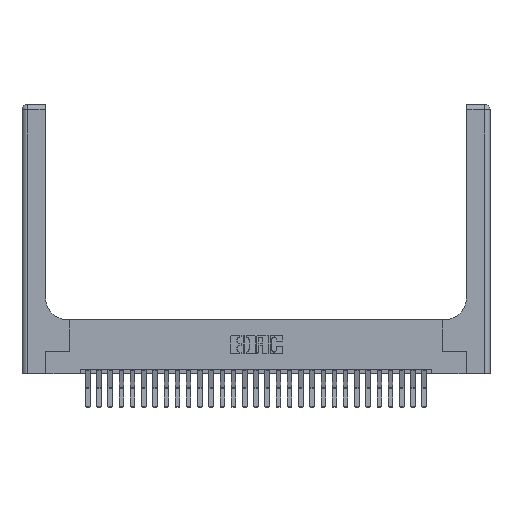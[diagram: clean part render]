
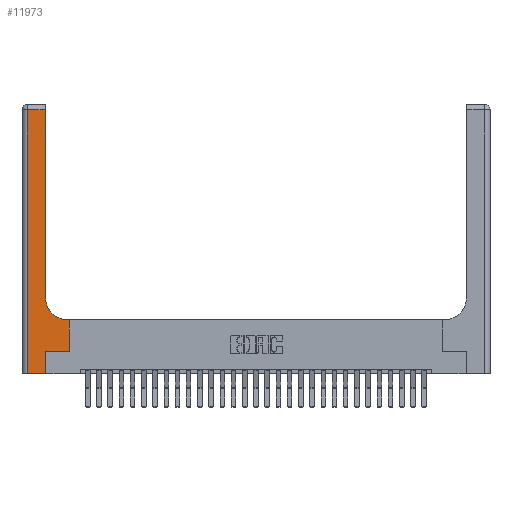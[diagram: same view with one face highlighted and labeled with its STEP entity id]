
A CAD part, top view. The second image highlights one B-rep face of the part: STEP entity #11973.
In plain terms, the highlighted planar face has unit normal (0, 0, 1).
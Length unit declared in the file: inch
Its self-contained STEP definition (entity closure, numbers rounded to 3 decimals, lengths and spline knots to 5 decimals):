
#353 = CARTESIAN_POINT ( 'NONE',  ( 0.26, 0.85, 0.37 ) ) ;
#372 = VECTOR ( 'NONE', #5949, 39.37008 ) ;
#550 = VECTOR ( 'NONE', #26776, 39.37008 ) ;
#918 = DIRECTION ( 'NONE',  ( 0., 1., 0. ) ) ;
#1443 = VECTOR ( 'NONE', #22164, 39.37008 ) ;
#1500 = CARTESIAN_POINT ( 'NONE',  ( 0.528, 0.6, 0.37 ) ) ;
#1703 = CARTESIAN_POINT ( 'NONE',  ( 0.06, 3., 0.37 ) ) ;
#2152 = VECTOR ( 'NONE', #21923, 39.37008 ) ;
#2194 = VERTEX_POINT ( 'NONE', #26470 ) ;
#2475 = VECTOR ( 'NONE', #24193, 39.37008 ) ;
#2741 = FACE_OUTER_BOUND ( 'NONE', #7920, .T. ) ;
#2832 = CARTESIAN_POINT ( 'NONE',  ( 0.528, 0.25, 0.37 ) ) ;
#2916 = CARTESIAN_POINT ( 'NONE',  ( 0., 3., 0.37 ) ) ;
#3122 = LINE ( 'NONE', #1703, #550 ) ;
#3288 = LINE ( 'NONE', #10048, #372 ) ;
#3706 = DIRECTION ( 'NONE',  ( 1., 0., 0. ) ) ;
#3867 = DIRECTION ( 'NONE',  ( 0., 1., 0. ) ) ;
#4148 = VERTEX_POINT ( 'NONE', #10153 ) ;
#4173 = EDGE_CURVE ( 'NONE', #6302, #22928, #17925, .T. ) ;
#4241 = ORIENTED_EDGE ( 'NONE', *, *, #5805, .T. ) ;
#5735 = EDGE_CURVE ( 'NONE', #17416, #2194, #3122, .T. ) ;
#5805 = EDGE_CURVE ( 'NONE', #22795, #18878, #3288, .T. ) ;
#5823 = ORIENTED_EDGE ( 'NONE', *, *, #12052, .T. ) ;
#5924 = CARTESIAN_POINT ( 'NONE',  ( 0.265, 0., 0.37 ) ) ;
#5949 = DIRECTION ( 'NONE',  ( 1., 0., 0. ) ) ;
#6302 = VERTEX_POINT ( 'NONE', #353 ) ;
#6583 = CIRCLE ( 'NONE', #9615, 0.25 ) ;
#6872 = AXIS2_PLACEMENT_3D ( 'NONE', #2916, #17499, #7215 ) ;
#7215 = DIRECTION ( 'NONE',  ( -1., 0., 0. ) ) ;
#7342 = CARTESIAN_POINT ( 'NONE',  ( 0.265, 0., 0.37 ) ) ;
#7920 = EDGE_LOOP ( 'NONE', ( #12587, #22412, #9055, #22798, #24188, #4241, #15621, #5823, #16695 ) ) ;
#7940 = CARTESIAN_POINT ( 'NONE',  ( 0.51, 0.85, 0.37 ) ) ;
#8117 = DIRECTION ( 'NONE',  ( 0., 0., -1. ) ) ;
#8351 = CARTESIAN_POINT ( 'NONE',  ( 0.265, 0.25, 0.37 ) ) ;
#9055 = ORIENTED_EDGE ( 'NONE', *, *, #5735, .T. ) ;
#9591 = EDGE_CURVE ( 'NONE', #4148, #6302, #6583, .T. ) ;
#9615 = AXIS2_PLACEMENT_3D ( 'NONE', #7940, #8117, #22510 ) ;
#10048 = CARTESIAN_POINT ( 'NONE',  ( 0.265, 0.25, 0.37 ) ) ;
#10153 = CARTESIAN_POINT ( 'NONE',  ( 0.51, 0.6, 0.37 ) ) ;
#11111 = EDGE_CURVE ( 'NONE', #18878, #23563, #21078, .T. ) ;
#11221 = EDGE_CURVE ( 'NONE', #12202, #22795, #18783, .T. ) ;
#11266 = CARTESIAN_POINT ( 'NONE',  ( 0.06, 2.94, 0.37 ) ) ;
#11388 = VECTOR ( 'NONE', #3706, 39.37008 ) ;
#11712 = LINE ( 'NONE', #11822, #11388 ) ;
#11822 = CARTESIAN_POINT ( 'NONE',  ( 0., 0., 0.37 ) ) ;
#11973 = ADVANCED_FACE ( 'NONE', ( #2741 ), #23725, .F. ) ;
#12052 = EDGE_CURVE ( 'NONE', #23563, #4148, #14469, .T. ) ;
#12202 = VERTEX_POINT ( 'NONE', #5924 ) ;
#12587 = ORIENTED_EDGE ( 'NONE', *, *, #4173, .T. ) ;
#12695 = CARTESIAN_POINT ( 'NONE',  ( 0.26, 2.94, 0.37 ) ) ;
#13572 = CARTESIAN_POINT ( 'NONE',  ( 0.26, 0.6, 0.37 ) ) ;
#14469 = LINE ( 'NONE', #13572, #1443 ) ;
#15368 = EDGE_CURVE ( 'NONE', #2194, #12202, #11712, .T. ) ;
#15621 = ORIENTED_EDGE ( 'NONE', *, *, #11111, .T. ) ;
#16325 = CARTESIAN_POINT ( 'NONE',  ( 0.26, 3., 0.37 ) ) ;
#16695 = ORIENTED_EDGE ( 'NONE', *, *, #9591, .T. ) ;
#17416 = VERTEX_POINT ( 'NONE', #11266 ) ;
#17499 = DIRECTION ( 'NONE',  ( 0., 0., -1. ) ) ;
#17925 = LINE ( 'NONE', #16325, #25109 ) ;
#18783 = LINE ( 'NONE', #7342, #2152 ) ;
#18878 = VERTEX_POINT ( 'NONE', #2832 ) ;
#20080 = CARTESIAN_POINT ( 'NONE',  ( 0., 2.94, 0.37 ) ) ;
#21078 = LINE ( 'NONE', #21618, #23361 ) ;
#21501 = EDGE_CURVE ( 'NONE', #22928, #17416, #26614, .T. ) ;
#21618 = CARTESIAN_POINT ( 'NONE',  ( 0.528, 0.25, 0.37 ) ) ;
#21923 = DIRECTION ( 'NONE',  ( 0., 1., 0. ) ) ;
#22164 = DIRECTION ( 'NONE',  ( -1., 0., 0. ) ) ;
#22412 = ORIENTED_EDGE ( 'NONE', *, *, #21501, .T. ) ;
#22510 = DIRECTION ( 'NONE',  ( 1., 0., 0. ) ) ;
#22795 = VERTEX_POINT ( 'NONE', #8351 ) ;
#22798 = ORIENTED_EDGE ( 'NONE', *, *, #15368, .T. ) ;
#22928 = VERTEX_POINT ( 'NONE', #12695 ) ;
#23361 = VECTOR ( 'NONE', #918, 39.37008 ) ;
#23563 = VERTEX_POINT ( 'NONE', #1500 ) ;
#23725 = PLANE ( 'NONE',  #6872 ) ;
#24188 = ORIENTED_EDGE ( 'NONE', *, *, #11221, .T. ) ;
#24193 = DIRECTION ( 'NONE',  ( -1., 0., 0. ) ) ;
#25109 = VECTOR ( 'NONE', #3867, 39.37008 ) ;
#26470 = CARTESIAN_POINT ( 'NONE',  ( 0.06, 0., 0.37 ) ) ;
#26614 = LINE ( 'NONE', #20080, #2475 ) ;
#26776 = DIRECTION ( 'NONE',  ( 0., -1., 0. ) ) ;
